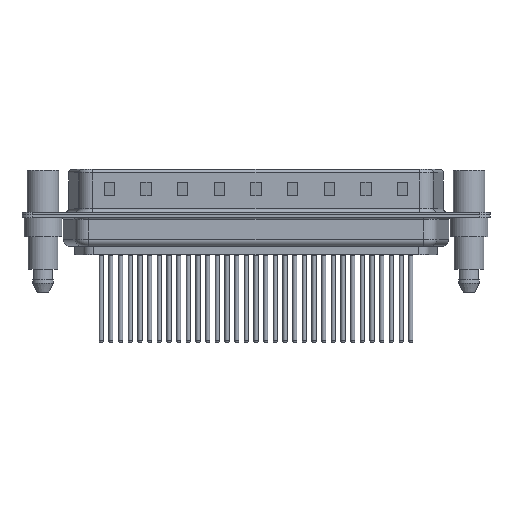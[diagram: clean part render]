
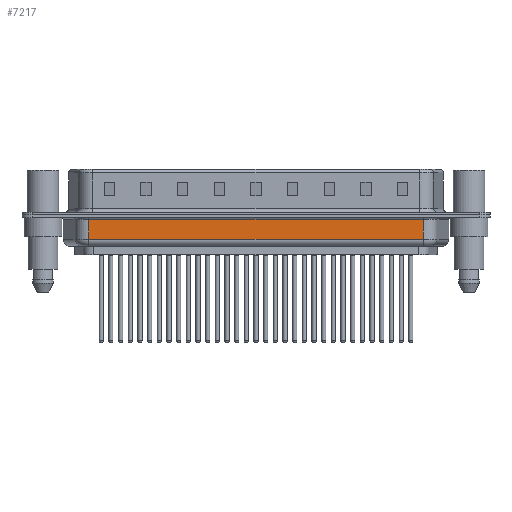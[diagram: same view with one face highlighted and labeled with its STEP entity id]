
A CAD part, front view. The second image highlights one B-rep face of the part: STEP entity #7217.
In plain terms, the highlighted planar face has unit normal (0, -1, 0).
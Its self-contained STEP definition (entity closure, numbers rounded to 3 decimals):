
#1539 = VERTEX_POINT ( 'NONE', #17072 ) ;
#1760 = VECTOR ( 'NONE', #17326, 1000. ) ;
#1847 = EDGE_CURVE ( 'NONE', #7813, #12331, #18562, .T. ) ;
#2064 = EDGE_CURVE ( 'NONE', #7813, #1539, #29064, .T. ) ;
#2252 = ORIENTED_EDGE ( 'NONE', *, *, #7442, .T. ) ;
#2334 = VERTEX_POINT ( 'NONE', #20327 ) ;
#3942 = DIRECTION ( 'NONE',  ( 0., 1., 0. ) ) ;
#4728 = CARTESIAN_POINT ( 'NONE',  ( 6.575, -6.75, -4.5 ) ) ;
#5985 = EDGE_LOOP ( 'NONE', ( #25018, #22540, #21997, #2252 ) ) ;
#7101 = EDGE_CURVE ( 'NONE', #1539, #2334, #19439, .T. ) ;
#7217 = ADVANCED_FACE ( 'NONE', ( #24388 ), #8909, .F. ) ;
#7442 = EDGE_CURVE ( 'NONE', #2334, #12331, #9949, .T. ) ;
#7813 = VERTEX_POINT ( 'NONE', #14123 ) ;
#8909 = PLANE ( 'NONE',  #26512 ) ;
#9949 = LINE ( 'NONE', #28145, #25244 ) ;
#12331 = VERTEX_POINT ( 'NONE', #25712 ) ;
#12683 = VECTOR ( 'NONE', #13748, 1000. ) ;
#13748 = DIRECTION ( 'NONE',  ( 0., 0., 1. ) ) ;
#14123 = CARTESIAN_POINT ( 'NONE',  ( 6.575, -6.75, -3.5 ) ) ;
#17072 = CARTESIAN_POINT ( 'NONE',  ( 54.425, -6.75, -3.5 ) ) ;
#17188 = CARTESIAN_POINT ( 'NONE',  ( 54.425, -6.75, -4.5 ) ) ;
#17326 = DIRECTION ( 'NONE',  ( 0., 0., 1. ) ) ;
#17482 = DIRECTION ( 'NONE',  ( 0., 0., 1. ) ) ;
#18562 = LINE ( 'NONE', #4728, #12683 ) ;
#19439 = LINE ( 'NONE', #17188, #1760 ) ;
#20327 = CARTESIAN_POINT ( 'NONE',  ( 54.425, -6.75, -0.65 ) ) ;
#21997 = ORIENTED_EDGE ( 'NONE', *, *, #7101, .T. ) ;
#22295 = DIRECTION ( 'NONE',  ( 1., 0., 0. ) ) ;
#22540 = ORIENTED_EDGE ( 'NONE', *, *, #2064, .T. ) ;
#22585 = CARTESIAN_POINT ( 'NONE',  ( 6.575, -6.75, -4.5 ) ) ;
#24061 = DIRECTION ( 'NONE',  ( -1., 0., 0. ) ) ;
#24388 = FACE_OUTER_BOUND ( 'NONE', #5985, .T. ) ;
#25018 = ORIENTED_EDGE ( 'NONE', *, *, #1847, .F. ) ;
#25244 = VECTOR ( 'NONE', #24061, 1000. ) ;
#25712 = CARTESIAN_POINT ( 'NONE',  ( 6.575, -6.75, -0.65 ) ) ;
#26162 = VECTOR ( 'NONE', #22295, 1000. ) ;
#26512 = AXIS2_PLACEMENT_3D ( 'NONE', #22585, #3942, #17482 ) ;
#28145 = CARTESIAN_POINT ( 'NONE',  ( 6.575, -6.75, -0.65 ) ) ;
#28623 = CARTESIAN_POINT ( 'NONE',  ( 6.575, -6.75, -3.5 ) ) ;
#29064 = LINE ( 'NONE', #28623, #26162 ) ;
